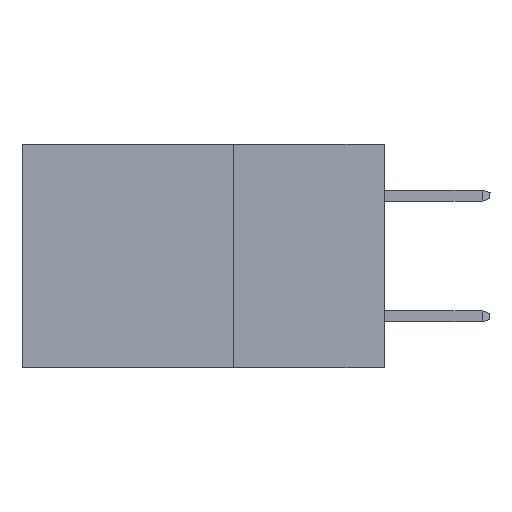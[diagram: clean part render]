
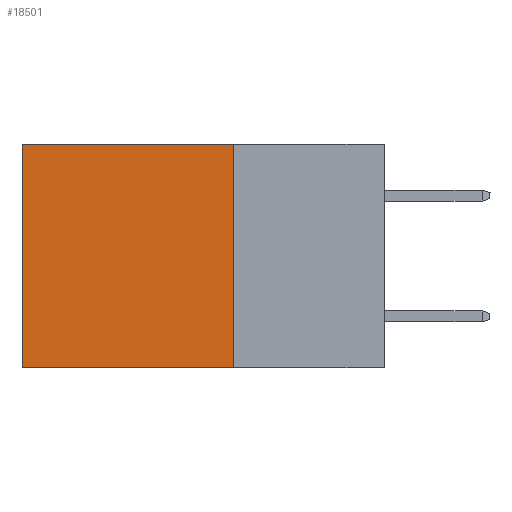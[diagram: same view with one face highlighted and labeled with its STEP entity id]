
A CAD part, left-side view. The second image highlights one B-rep face of the part: STEP entity #18501.
In plain terms, the highlighted planar face has unit normal (-1, 0, 0).
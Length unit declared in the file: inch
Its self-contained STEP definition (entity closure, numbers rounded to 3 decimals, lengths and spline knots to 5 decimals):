
#63 = EDGE_CURVE ( 'NONE', #4026, #10184, #4127, .T. ) ;
#617 = EDGE_LOOP ( 'NONE', ( #2178, #12241, #18431, #5284 ) ) ;
#1534 = FACE_OUTER_BOUND ( 'NONE', #617, .T. ) ;
#2178 = ORIENTED_EDGE ( 'NONE', *, *, #5081, .T. ) ;
#2945 = VECTOR ( 'NONE', #15167, 39.37008 ) ;
#4026 = VERTEX_POINT ( 'NONE', #11792 ) ;
#4119 = EDGE_CURVE ( 'NONE', #21248, #4026, #18817, .T. ) ;
#4127 = LINE ( 'NONE', #14963, #2945 ) ;
#5074 = CARTESIAN_POINT ( 'NONE',  ( 0.2615, 0.6, 0. ) ) ;
#5081 = EDGE_CURVE ( 'NONE', #17712, #10184, #18929, .T. ) ;
#5284 = ORIENTED_EDGE ( 'NONE', *, *, #19386, .T. ) ;
#7023 = DIRECTION ( 'NONE',  ( 0., 0., -1. ) ) ;
#7257 = CARTESIAN_POINT ( 'NONE',  ( 0.2615, 0.6, -0.37 ) ) ;
#8937 = DIRECTION ( 'NONE',  ( 0., 0., -1. ) ) ;
#9020 = CARTESIAN_POINT ( 'NONE',  ( 0.2615, 0.25, -0.37 ) ) ;
#10184 = VERTEX_POINT ( 'NONE', #7257 ) ;
#10381 = LINE ( 'NONE', #22084, #20138 ) ;
#11101 = DIRECTION ( 'NONE',  ( 0., 1., 0. ) ) ;
#11792 = CARTESIAN_POINT ( 'NONE',  ( 0.2615, 0.25, -0.37 ) ) ;
#12241 = ORIENTED_EDGE ( 'NONE', *, *, #63, .F. ) ;
#14744 = DIRECTION ( 'NONE',  ( 0., 0., -1. ) ) ;
#14858 = CARTESIAN_POINT ( 'NONE',  ( 0.2615, 0.6, -0.37 ) ) ;
#14963 = CARTESIAN_POINT ( 'NONE',  ( 0.2615, 0.25, -0.37 ) ) ;
#15167 = DIRECTION ( 'NONE',  ( 0., 1., 0. ) ) ;
#15755 = CARTESIAN_POINT ( 'NONE',  ( 0.2615, 0.25, 0. ) ) ;
#16136 = PLANE ( 'NONE',  #20859 ) ;
#17712 = VERTEX_POINT ( 'NONE', #5074 ) ;
#17973 = DIRECTION ( 'NONE',  ( 1., 0., 0. ) ) ;
#18431 = ORIENTED_EDGE ( 'NONE', *, *, #4119, .F. ) ;
#18501 = ADVANCED_FACE ( 'NONE', ( #1534 ), #16136, .F. ) ;
#18817 = LINE ( 'NONE', #9020, #19404 ) ;
#18929 = LINE ( 'NONE', #14858, #23167 ) ;
#19386 = EDGE_CURVE ( 'NONE', #21248, #17712, #10381, .T. ) ;
#19404 = VECTOR ( 'NONE', #8937, 39.37008 ) ;
#20138 = VECTOR ( 'NONE', #11101, 39.37008 ) ;
#20859 = AXIS2_PLACEMENT_3D ( 'NONE', #23358, #17973, #7023 ) ;
#21248 = VERTEX_POINT ( 'NONE', #15755 ) ;
#22084 = CARTESIAN_POINT ( 'NONE',  ( 0.2615, 0.25, 0. ) ) ;
#23167 = VECTOR ( 'NONE', #14744, 39.37008 ) ;
#23358 = CARTESIAN_POINT ( 'NONE',  ( 0.2615, 0.25, -0.37 ) ) ;
